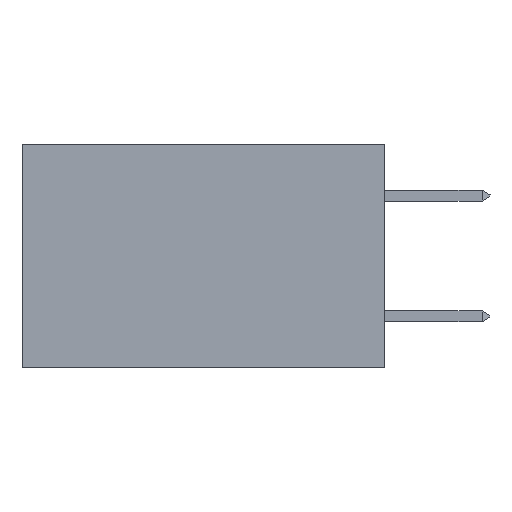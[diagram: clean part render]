
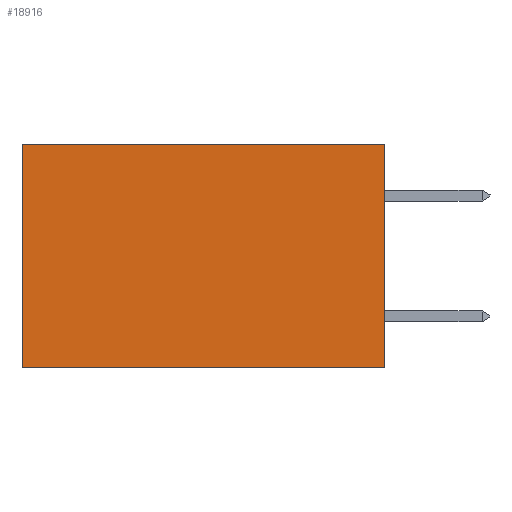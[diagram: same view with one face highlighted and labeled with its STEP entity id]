
A CAD part, left-side view. The second image highlights one B-rep face of the part: STEP entity #18916.
In plain terms, the highlighted planar face has unit normal (-1, 0, 0).
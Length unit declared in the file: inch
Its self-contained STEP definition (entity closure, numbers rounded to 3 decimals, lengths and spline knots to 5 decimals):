
#637 = CARTESIAN_POINT ( 'NONE',  ( 0.2875, 0.6, 0. ) ) ;
#2066 = DIRECTION ( 'NONE',  ( 1., 0., 0. ) ) ;
#4375 = ORIENTED_EDGE ( 'NONE', *, *, #23918, .T. ) ;
#4409 = FACE_OUTER_BOUND ( 'NONE', #17126, .T. ) ;
#5035 = VECTOR ( 'NONE', #13974, 39.37008 ) ;
#6286 = LINE ( 'NONE', #13495, #14163 ) ;
#7219 = VERTEX_POINT ( 'NONE', #637 ) ;
#8123 = LINE ( 'NONE', #24182, #37411 ) ;
#8483 = EDGE_CURVE ( 'NONE', #27353, #32992, #12940, .T. ) ;
#10437 = AXIS2_PLACEMENT_3D ( 'NONE', #22646, #2066, #22763 ) ;
#10496 = DIRECTION ( 'NONE',  ( 0., 0., -1. ) ) ;
#12544 = EDGE_CURVE ( 'NONE', #7219, #32992, #28592, .T. ) ;
#12940 = LINE ( 'NONE', #37184, #5035 ) ;
#13495 = CARTESIAN_POINT ( 'NONE',  ( 0.2875, 0., 0. ) ) ;
#13747 = PLANE ( 'NONE',  #10437 ) ;
#13795 = ORIENTED_EDGE ( 'NONE', *, *, #12544, .T. ) ;
#13974 = DIRECTION ( 'NONE',  ( 0., 1., 0. ) ) ;
#14163 = VECTOR ( 'NONE', #10496, 39.37008 ) ;
#15044 = DIRECTION ( 'NONE',  ( 0., 0., -1. ) ) ;
#17126 = EDGE_LOOP ( 'NONE', ( #13795, #37976, #18645, #4375 ) ) ;
#18645 = ORIENTED_EDGE ( 'NONE', *, *, #18823, .F. ) ;
#18823 = EDGE_CURVE ( 'NONE', #26394, #27353, #6286, .T. ) ;
#18916 = ADVANCED_FACE ( 'NONE', ( #4409 ), #13747, .F. ) ;
#22646 = CARTESIAN_POINT ( 'NONE',  ( 0.2875, 0., 0. ) ) ;
#22763 = DIRECTION ( 'NONE',  ( 0., 0., -1. ) ) ;
#22977 = CARTESIAN_POINT ( 'NONE',  ( 0.2875, 0.6, -0.37 ) ) ;
#23918 = EDGE_CURVE ( 'NONE', #26394, #7219, #8123, .T. ) ;
#24162 = CARTESIAN_POINT ( 'NONE',  ( 0.2875, 0., 0. ) ) ;
#24182 = CARTESIAN_POINT ( 'NONE',  ( 0.2875, 0., 0. ) ) ;
#26394 = VERTEX_POINT ( 'NONE', #24162 ) ;
#27353 = VERTEX_POINT ( 'NONE', #31056 ) ;
#28592 = LINE ( 'NONE', #32514, #36318 ) ;
#31056 = CARTESIAN_POINT ( 'NONE',  ( 0.2875, 0., -0.37 ) ) ;
#32514 = CARTESIAN_POINT ( 'NONE',  ( 0.2875, 0.6, 0. ) ) ;
#32992 = VERTEX_POINT ( 'NONE', #22977 ) ;
#35846 = DIRECTION ( 'NONE',  ( 0., 1., 0. ) ) ;
#36318 = VECTOR ( 'NONE', #15044, 39.37008 ) ;
#37184 = CARTESIAN_POINT ( 'NONE',  ( 0.2875, 0., -0.37 ) ) ;
#37411 = VECTOR ( 'NONE', #35846, 39.37008 ) ;
#37976 = ORIENTED_EDGE ( 'NONE', *, *, #8483, .F. ) ;
